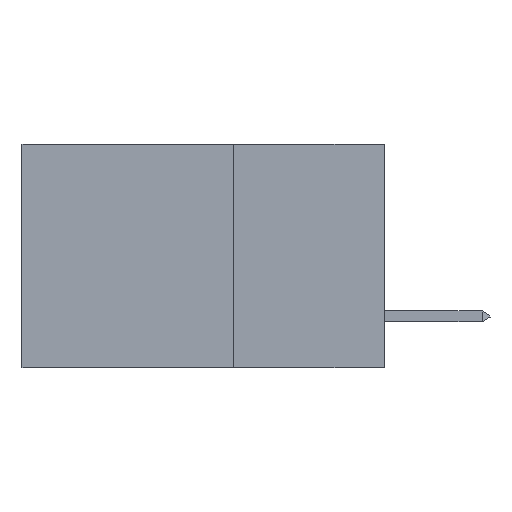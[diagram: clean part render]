
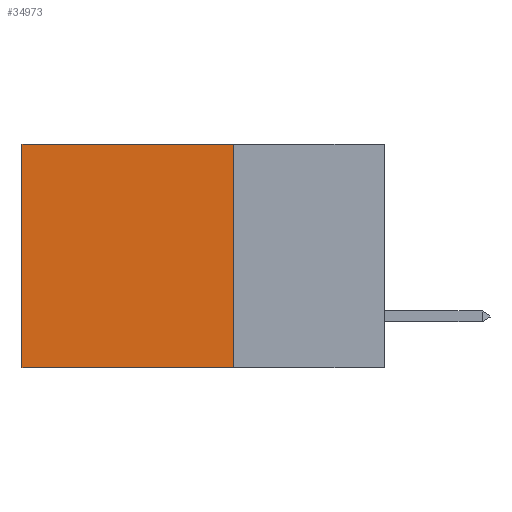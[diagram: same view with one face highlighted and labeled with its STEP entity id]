
A CAD part, left-side view. The second image highlights one B-rep face of the part: STEP entity #34973.
In plain terms, the highlighted planar face has unit normal (-1, 0, 0).
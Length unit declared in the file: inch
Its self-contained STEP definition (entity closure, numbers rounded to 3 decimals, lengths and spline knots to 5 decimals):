
#378 = EDGE_CURVE ( 'NONE', #24255, #16544, #31083, .T. ) ;
#684 = EDGE_CURVE ( 'NONE', #8923, #23730, #12466, .T. ) ;
#934 = LINE ( 'NONE', #15189, #37155 ) ;
#3424 = DIRECTION ( 'NONE',  ( 0., 0., -1. ) ) ;
#4653 = EDGE_CURVE ( 'NONE', #16544, #23730, #27463, .T. ) ;
#8545 = PLANE ( 'NONE',  #23927 ) ;
#8829 = VECTOR ( 'NONE', #9855, 39.37008 ) ;
#8923 = VERTEX_POINT ( 'NONE', #11611 ) ;
#9855 = DIRECTION ( 'NONE',  ( 0., 1., 0. ) ) ;
#9940 = EDGE_CURVE ( 'NONE', #24255, #8923, #934, .T. ) ;
#10683 = CARTESIAN_POINT ( 'NONE',  ( 0.2875, 0.6, -0.37 ) ) ;
#11573 = CARTESIAN_POINT ( 'NONE',  ( 0.2875, 0.25, 0. ) ) ;
#11611 = CARTESIAN_POINT ( 'NONE',  ( 0.2875, 0.25, -0.37 ) ) ;
#12328 = DIRECTION ( 'NONE',  ( 1., 0., 0. ) ) ;
#12466 = LINE ( 'NONE', #42564, #22759 ) ;
#13008 = VECTOR ( 'NONE', #35617, 39.37008 ) ;
#15189 = CARTESIAN_POINT ( 'NONE',  ( 0.2875, 0.25, 0. ) ) ;
#15328 = DIRECTION ( 'NONE',  ( 0., 0., -1. ) ) ;
#16544 = VERTEX_POINT ( 'NONE', #40240 ) ;
#18391 = ORIENTED_EDGE ( 'NONE', *, *, #9940, .F. ) ;
#21699 = ORIENTED_EDGE ( 'NONE', *, *, #4653, .T. ) ;
#22759 = VECTOR ( 'NONE', #26489, 39.37008 ) ;
#22945 = ORIENTED_EDGE ( 'NONE', *, *, #684, .F. ) ;
#23730 = VERTEX_POINT ( 'NONE', #10683 ) ;
#23927 = AXIS2_PLACEMENT_3D ( 'NONE', #35180, #12328, #15328 ) ;
#24255 = VERTEX_POINT ( 'NONE', #11573 ) ;
#26489 = DIRECTION ( 'NONE',  ( 0., 1., 0. ) ) ;
#27337 = CARTESIAN_POINT ( 'NONE',  ( 0.2875, 0.6, 0. ) ) ;
#27463 = LINE ( 'NONE', #27337, #13008 ) ;
#28917 = ORIENTED_EDGE ( 'NONE', *, *, #378, .T. ) ;
#31083 = LINE ( 'NONE', #36179, #8829 ) ;
#32619 = FACE_OUTER_BOUND ( 'NONE', #34495, .T. ) ;
#34495 = EDGE_LOOP ( 'NONE', ( #21699, #22945, #18391, #28917 ) ) ;
#34973 = ADVANCED_FACE ( 'NONE', ( #32619 ), #8545, .F. ) ;
#35180 = CARTESIAN_POINT ( 'NONE',  ( 0.2875, 0.25, 0. ) ) ;
#35617 = DIRECTION ( 'NONE',  ( 0., 0., -1. ) ) ;
#36179 = CARTESIAN_POINT ( 'NONE',  ( 0.2875, 0.25, 0. ) ) ;
#37155 = VECTOR ( 'NONE', #3424, 39.37008 ) ;
#40240 = CARTESIAN_POINT ( 'NONE',  ( 0.2875, 0.6, 0. ) ) ;
#42564 = CARTESIAN_POINT ( 'NONE',  ( 0.2875, 0.25, -0.37 ) ) ;
